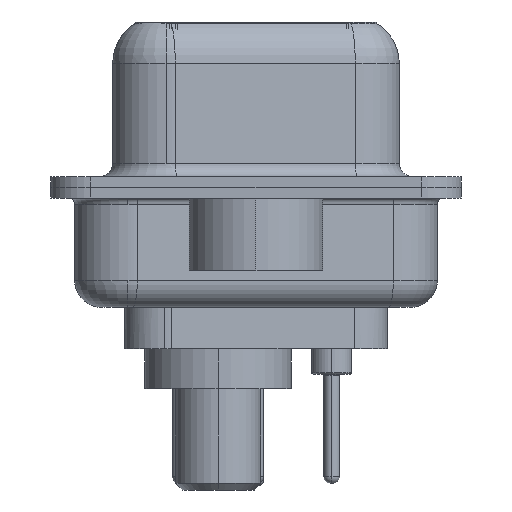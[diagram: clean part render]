
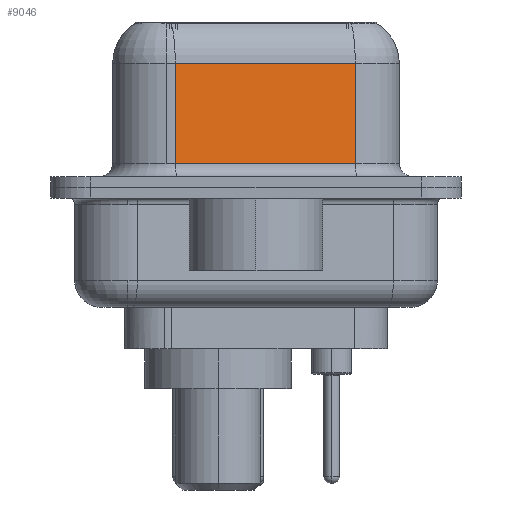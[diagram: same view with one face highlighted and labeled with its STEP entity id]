
A CAD part, left-side view. The second image highlights one B-rep face of the part: STEP entity #9046.
In plain terms, the highlighted planar face has unit normal (-0.985, -0.174, 0).
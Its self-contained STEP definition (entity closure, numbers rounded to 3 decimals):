
#84 = CARTESIAN_POINT ( 'NONE',  ( 5.621, -3.722, 6.4 ) ) ;
#320 = EDGE_CURVE ( 'NONE', #10695, #7243, #30889, .T. ) ;
#601 = CARTESIAN_POINT ( 'NONE',  ( 4.43, 3.028, 4.65 ) ) ;
#731 = EDGE_LOOP ( 'NONE', ( #17070, #18104, #22362, #28777 ) ) ;
#4418 = CARTESIAN_POINT ( 'NONE',  ( 5.621, -3.722, 0.9 ) ) ;
#6738 = DIRECTION ( 'NONE',  ( 0.174, -0.985, 0. ) ) ;
#7243 = VERTEX_POINT ( 'NONE', #21860 ) ;
#7287 = AXIS2_PLACEMENT_3D ( 'NONE', #16252, #21624, #29546 ) ;
#7752 = LINE ( 'NONE', #84, #14686 ) ;
#7961 = VECTOR ( 'NONE', #33876, 1000. ) ;
#8032 = EDGE_CURVE ( 'NONE', #32593, #10695, #29605, .T. ) ;
#8461 = PLANE ( 'NONE',  #7287 ) ;
#9046 = ADVANCED_FACE ( 'NONE', ( #16698 ), #8461, .F. ) ;
#10264 = CARTESIAN_POINT ( 'NONE',  ( 4.43, 3.028, 6.4 ) ) ;
#10695 = VERTEX_POINT ( 'NONE', #601 ) ;
#13059 = VECTOR ( 'NONE', #6738, 1000. ) ;
#14686 = VECTOR ( 'NONE', #20691, 1000. ) ;
#15866 = VERTEX_POINT ( 'NONE', #4418 ) ;
#16252 = CARTESIAN_POINT ( 'NONE',  ( 5.621, -3.722, 6.4 ) ) ;
#16698 = FACE_OUTER_BOUND ( 'NONE', #731, .T. ) ;
#16837 = LINE ( 'NONE', #22359, #13059 ) ;
#17070 = ORIENTED_EDGE ( 'NONE', *, *, #30278, .F. ) ;
#18030 = DIRECTION ( 'NONE',  ( -0.174, 0.985, 0. ) ) ;
#18104 = ORIENTED_EDGE ( 'NONE', *, *, #8032, .T. ) ;
#19375 = VECTOR ( 'NONE', #18030, 1000. ) ;
#20691 = DIRECTION ( 'NONE',  ( 0., 0., -1. ) ) ;
#21624 = DIRECTION ( 'NONE',  ( 0.985, 0.174, 0. ) ) ;
#21860 = CARTESIAN_POINT ( 'NONE',  ( 4.43, 3.028, 0.9 ) ) ;
#22359 = CARTESIAN_POINT ( 'NONE',  ( 5.621, -3.722, 0.9 ) ) ;
#22362 = ORIENTED_EDGE ( 'NONE', *, *, #320, .T. ) ;
#28777 = ORIENTED_EDGE ( 'NONE', *, *, #28876, .T. ) ;
#28876 = EDGE_CURVE ( 'NONE', #7243, #15866, #16837, .T. ) ;
#29546 = DIRECTION ( 'NONE',  ( -0.174, 0.985, 0. ) ) ;
#29605 = LINE ( 'NONE', #31077, #19375 ) ;
#30278 = EDGE_CURVE ( 'NONE', #32593, #15866, #7752, .T. ) ;
#30889 = LINE ( 'NONE', #10264, #7961 ) ;
#31077 = CARTESIAN_POINT ( 'NONE',  ( 5.621, -3.722, 4.65 ) ) ;
#31463 = CARTESIAN_POINT ( 'NONE',  ( 5.621, -3.722, 4.65 ) ) ;
#32593 = VERTEX_POINT ( 'NONE', #31463 ) ;
#33876 = DIRECTION ( 'NONE',  ( 0., 0., -1. ) ) ;
